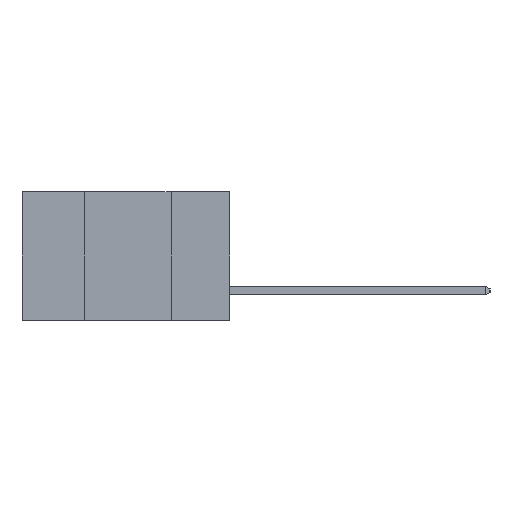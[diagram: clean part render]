
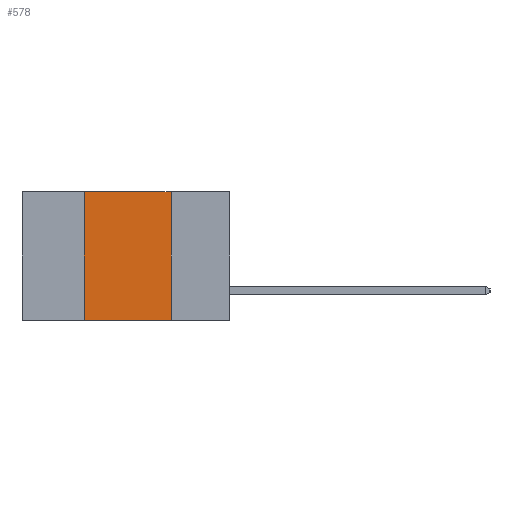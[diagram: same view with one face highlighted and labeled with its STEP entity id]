
A CAD part, left-side view. The second image highlights one B-rep face of the part: STEP entity #578.
In plain terms, the highlighted planar face has unit normal (-1, 0, 0).
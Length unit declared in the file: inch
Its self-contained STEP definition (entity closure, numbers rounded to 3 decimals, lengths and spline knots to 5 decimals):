
#175 = LINE ( 'NONE', #7711, #8411 ) ;
#578 = ADVANCED_FACE ( 'NONE', ( #4864 ), #8549, .F. ) ;
#1680 = ORIENTED_EDGE ( 'NONE', *, *, #8483, .F. ) ;
#1994 = DIRECTION ( 'NONE',  ( 0., 0., -1. ) ) ;
#3223 = EDGE_CURVE ( 'NONE', #18203, #9570, #175, .T. ) ;
#3708 = CARTESIAN_POINT ( 'NONE',  ( 0., 0.17, -0.37 ) ) ;
#4138 = LINE ( 'NONE', #4599, #11320 ) ;
#4400 = VECTOR ( 'NONE', #16238, 39.37008 ) ;
#4599 = CARTESIAN_POINT ( 'NONE',  ( 0., 0.42, 0. ) ) ;
#4864 = FACE_OUTER_BOUND ( 'NONE', #6000, .T. ) ;
#4935 = CARTESIAN_POINT ( 'NONE',  ( 0., 0.17, 0. ) ) ;
#5147 = ORIENTED_EDGE ( 'NONE', *, *, #6041, .F. ) ;
#5180 = AXIS2_PLACEMENT_3D ( 'NONE', #6180, #17739, #1994 ) ;
#5735 = CARTESIAN_POINT ( 'NONE',  ( 0., 0.17, 0. ) ) ;
#5798 = DIRECTION ( 'NONE',  ( 0., 0., -1. ) ) ;
#6000 = EDGE_LOOP ( 'NONE', ( #5147, #1680, #9858, #6554 ) ) ;
#6041 = EDGE_CURVE ( 'NONE', #15241, #9570, #18126, .T. ) ;
#6180 = CARTESIAN_POINT ( 'NONE',  ( 0., 0.6, 0. ) ) ;
#6554 = ORIENTED_EDGE ( 'NONE', *, *, #3223, .T. ) ;
#6580 = CARTESIAN_POINT ( 'NONE',  ( 0., 0.42, 0. ) ) ;
#7006 = VECTOR ( 'NONE', #5798, 39.37008 ) ;
#7711 = CARTESIAN_POINT ( 'NONE',  ( 0., 0.6, -0.37 ) ) ;
#8411 = VECTOR ( 'NONE', #13443, 39.37008 ) ;
#8473 = CARTESIAN_POINT ( 'NONE',  ( 0., 0.42, -0.37 ) ) ;
#8483 = EDGE_CURVE ( 'NONE', #8572, #15241, #12025, .T. ) ;
#8549 = PLANE ( 'NONE',  #5180 ) ;
#8572 = VERTEX_POINT ( 'NONE', #6580 ) ;
#9239 = CARTESIAN_POINT ( 'NONE',  ( 0., 0.6, 0. ) ) ;
#9570 = VERTEX_POINT ( 'NONE', #3708 ) ;
#9858 = ORIENTED_EDGE ( 'NONE', *, *, #15698, .F. ) ;
#11320 = VECTOR ( 'NONE', #17292, 39.37008 ) ;
#12025 = LINE ( 'NONE', #9239, #4400 ) ;
#13443 = DIRECTION ( 'NONE',  ( 0., -1., 0. ) ) ;
#15241 = VERTEX_POINT ( 'NONE', #4935 ) ;
#15698 = EDGE_CURVE ( 'NONE', #18203, #8572, #4138, .T. ) ;
#16238 = DIRECTION ( 'NONE',  ( 0., -1., 0. ) ) ;
#17292 = DIRECTION ( 'NONE',  ( 0., 0., 1. ) ) ;
#17739 = DIRECTION ( 'NONE',  ( 1., 0., 0. ) ) ;
#18126 = LINE ( 'NONE', #5735, #7006 ) ;
#18203 = VERTEX_POINT ( 'NONE', #8473 ) ;
